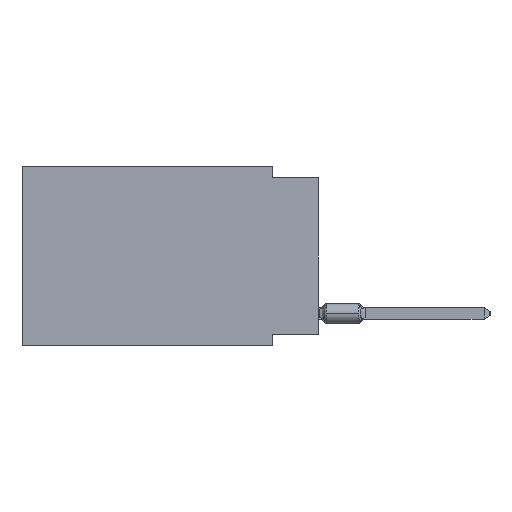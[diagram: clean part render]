
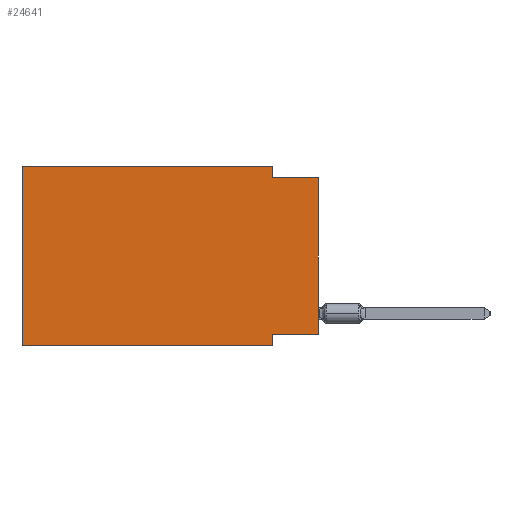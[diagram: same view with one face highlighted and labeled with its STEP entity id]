
A CAD part, left-side view. The second image highlights one B-rep face of the part: STEP entity #24641.
In plain terms, the highlighted planar face has unit normal (-1, 0, 0).
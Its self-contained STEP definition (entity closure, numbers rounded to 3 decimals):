
#495 = CARTESIAN_POINT ( 'NONE',  ( 0., 16.383, 0. ) ) ;
#914 = LINE ( 'NONE', #495, #21858 ) ;
#2971 = LINE ( 'NONE', #58559, #8347 ) ;
#7069 = VECTOR ( 'NONE', #10440, 1000. ) ;
#7399 = ORIENTED_EDGE ( 'NONE', *, *, #58027, .F. ) ;
#8347 = VECTOR ( 'NONE', #26815, 1000. ) ;
#8541 = DIRECTION ( 'NONE',  ( 0., 0., -1. ) ) ;
#10440 = DIRECTION ( 'NONE',  ( 0., 1., 0. ) ) ;
#11424 = CARTESIAN_POINT ( 'NONE',  ( 0., 16.383, 0. ) ) ;
#11839 = ORIENTED_EDGE ( 'NONE', *, *, #18809, .T. ) ;
#12442 = EDGE_CURVE ( 'NONE', #49752, #81091, #914, .T. ) ;
#13119 = VECTOR ( 'NONE', #19796, 1000. ) ;
#13996 = DIRECTION ( 'NONE',  ( 0., 0., -1. ) ) ;
#14496 = VECTOR ( 'NONE', #13996, 1000. ) ;
#16142 = LINE ( 'NONE', #35778, #58251 ) ;
#16288 = DIRECTION ( 'NONE',  ( 0., 0., -1. ) ) ;
#17208 = CARTESIAN_POINT ( 'NONE',  ( 0., 2.54, -9.271 ) ) ;
#18114 = EDGE_CURVE ( 'NONE', #75531, #81695, #33966, .T. ) ;
#18809 = EDGE_CURVE ( 'NONE', #49752, #70455, #82297, .T. ) ;
#19796 = DIRECTION ( 'NONE',  ( 0., 0., 1. ) ) ;
#20244 = CARTESIAN_POINT ( 'NONE',  ( 0., 2.54, -9.906 ) ) ;
#21858 = VECTOR ( 'NONE', #56921, 1000. ) ;
#23005 = VERTEX_POINT ( 'NONE', #17208 ) ;
#23152 = VERTEX_POINT ( 'NONE', #64782 ) ;
#24641 = ADVANCED_FACE ( 'NONE', ( #47627 ), #60568, .F. ) ;
#25679 = EDGE_LOOP ( 'NONE', ( #59619, #43343, #7399, #59715, #58543, #11839, #46733, #79097 ) ) ;
#26815 = DIRECTION ( 'NONE',  ( 0., -1., 0. ) ) ;
#27126 = AXIS2_PLACEMENT_3D ( 'NONE', #61406, #48033, #16288 ) ;
#31581 = CARTESIAN_POINT ( 'NONE',  ( 0., 2.54, -9.906 ) ) ;
#33966 = LINE ( 'NONE', #77448, #13119 ) ;
#34799 = VERTEX_POINT ( 'NONE', #80838 ) ;
#35778 = CARTESIAN_POINT ( 'NONE',  ( 0., 16.383, 0. ) ) ;
#40709 = CARTESIAN_POINT ( 'NONE',  ( 0., 2.54, 0. ) ) ;
#41442 = EDGE_CURVE ( 'NONE', #81091, #34799, #16142, .T. ) ;
#43025 = CARTESIAN_POINT ( 'NONE',  ( 0., 16.383, -9.906 ) ) ;
#43343 = ORIENTED_EDGE ( 'NONE', *, *, #80276, .F. ) ;
#46733 = ORIENTED_EDGE ( 'NONE', *, *, #61429, .F. ) ;
#47627 = FACE_OUTER_BOUND ( 'NONE', #25679, .T. ) ;
#47801 = LINE ( 'NONE', #40709, #70214 ) ;
#48033 = DIRECTION ( 'NONE',  ( 1., 0., 0. ) ) ;
#49752 = VERTEX_POINT ( 'NONE', #53527 ) ;
#52831 = LINE ( 'NONE', #20244, #14496 ) ;
#53527 = CARTESIAN_POINT ( 'NONE',  ( 0., 16.383, -9.906 ) ) ;
#55960 = LINE ( 'NONE', #73116, #7069 ) ;
#56921 = DIRECTION ( 'NONE',  ( 0., 0., 1. ) ) ;
#58027 = EDGE_CURVE ( 'NONE', #34799, #23152, #47801, .T. ) ;
#58251 = VECTOR ( 'NONE', #59607, 1000. ) ;
#58543 = ORIENTED_EDGE ( 'NONE', *, *, #12442, .F. ) ;
#58559 = CARTESIAN_POINT ( 'NONE',  ( 0., 0., -0.635 ) ) ;
#59607 = DIRECTION ( 'NONE',  ( 0., -1., 0. ) ) ;
#59619 = ORIENTED_EDGE ( 'NONE', *, *, #18114, .T. ) ;
#59715 = ORIENTED_EDGE ( 'NONE', *, *, #41442, .F. ) ;
#60568 = PLANE ( 'NONE',  #27126 ) ;
#61406 = CARTESIAN_POINT ( 'NONE',  ( 0., 16.383, 0. ) ) ;
#61429 = EDGE_CURVE ( 'NONE', #23005, #70455, #52831, .T. ) ;
#62692 = CARTESIAN_POINT ( 'NONE',  ( 0., 0., -0.635 ) ) ;
#62962 = CARTESIAN_POINT ( 'NONE',  ( 0., 0., -9.271 ) ) ;
#64782 = CARTESIAN_POINT ( 'NONE',  ( 0., 2.54, -0.635 ) ) ;
#68092 = DIRECTION ( 'NONE',  ( 0., -1., 0. ) ) ;
#70214 = VECTOR ( 'NONE', #8541, 1000. ) ;
#70455 = VERTEX_POINT ( 'NONE', #31581 ) ;
#73116 = CARTESIAN_POINT ( 'NONE',  ( 0., 0., -9.271 ) ) ;
#75531 = VERTEX_POINT ( 'NONE', #62962 ) ;
#77448 = CARTESIAN_POINT ( 'NONE',  ( 0., 0., 0. ) ) ;
#77601 = EDGE_CURVE ( 'NONE', #75531, #23005, #55960, .T. ) ;
#79097 = ORIENTED_EDGE ( 'NONE', *, *, #77601, .F. ) ;
#80276 = EDGE_CURVE ( 'NONE', #23152, #81695, #2971, .T. ) ;
#80838 = CARTESIAN_POINT ( 'NONE',  ( 0., 2.54, 0. ) ) ;
#81091 = VERTEX_POINT ( 'NONE', #11424 ) ;
#81220 = VECTOR ( 'NONE', #68092, 1000. ) ;
#81695 = VERTEX_POINT ( 'NONE', #62692 ) ;
#82297 = LINE ( 'NONE', #43025, #81220 ) ;
